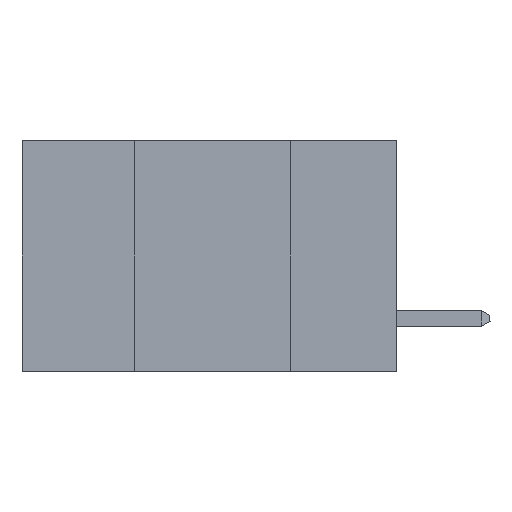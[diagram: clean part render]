
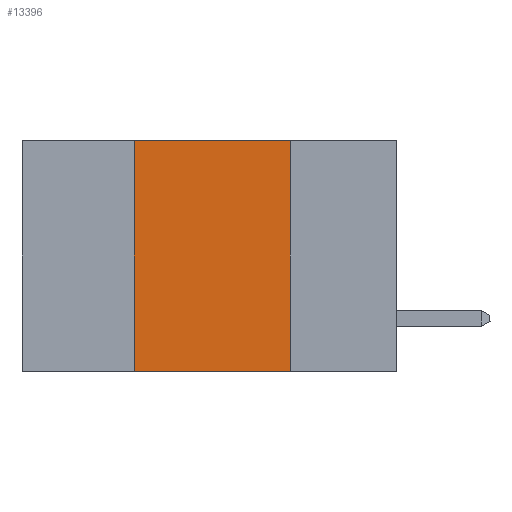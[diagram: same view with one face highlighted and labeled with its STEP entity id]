
A CAD part, left-side view. The second image highlights one B-rep face of the part: STEP entity #13396.
In plain terms, the highlighted planar face has unit normal (-1, 0, 0).
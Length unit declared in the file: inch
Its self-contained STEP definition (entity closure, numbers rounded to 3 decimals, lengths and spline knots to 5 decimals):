
#59 = LINE ( 'NONE', #626, #15693 ) ;
#314 = LINE ( 'NONE', #10184, #7683 ) ;
#399 = LINE ( 'NONE', #4879, #11413 ) ;
#626 = CARTESIAN_POINT ( 'NONE',  ( 0., 0.6, -0.37 ) ) ;
#2747 = DIRECTION ( 'NONE',  ( 0., -1., 0. ) ) ;
#3220 = CARTESIAN_POINT ( 'NONE',  ( 0., 0.42, -0.37 ) ) ;
#3722 = DIRECTION ( 'NONE',  ( 0., 0., 1. ) ) ;
#4752 = ORIENTED_EDGE ( 'NONE', *, *, #6087, .F. ) ;
#4879 = CARTESIAN_POINT ( 'NONE',  ( 0., 0.42, 0. ) ) ;
#4903 = VERTEX_POINT ( 'NONE', #10599 ) ;
#5265 = DIRECTION ( 'NONE',  ( 0., 0., -1. ) ) ;
#6087 = EDGE_CURVE ( 'NONE', #4903, #14718, #9009, .T. ) ;
#6720 = EDGE_LOOP ( 'NONE', ( #4752, #11530, #15313, #12016 ) ) ;
#7683 = VECTOR ( 'NONE', #2747, 39.37008 ) ;
#7796 = FACE_OUTER_BOUND ( 'NONE', #6720, .T. ) ;
#7815 = CARTESIAN_POINT ( 'NONE',  ( 0., 0.6, 0. ) ) ;
#8796 = CARTESIAN_POINT ( 'NONE',  ( 0., 0.17, -0.37 ) ) ;
#8860 = VERTEX_POINT ( 'NONE', #9410 ) ;
#9009 = LINE ( 'NONE', #13915, #10018 ) ;
#9224 = EDGE_CURVE ( 'NONE', #9664, #8860, #399, .T. ) ;
#9270 = DIRECTION ( 'NONE',  ( 0., -1., 0. ) ) ;
#9410 = CARTESIAN_POINT ( 'NONE',  ( 0., 0.42, 0. ) ) ;
#9664 = VERTEX_POINT ( 'NONE', #3220 ) ;
#9814 = AXIS2_PLACEMENT_3D ( 'NONE', #7815, #15173, #11510 ) ;
#10018 = VECTOR ( 'NONE', #5265, 39.37008 ) ;
#10184 = CARTESIAN_POINT ( 'NONE',  ( 0., 0.6, 0. ) ) ;
#10599 = CARTESIAN_POINT ( 'NONE',  ( 0., 0.17, 0. ) ) ;
#11131 = EDGE_CURVE ( 'NONE', #8860, #4903, #314, .T. ) ;
#11413 = VECTOR ( 'NONE', #3722, 39.37008 ) ;
#11510 = DIRECTION ( 'NONE',  ( 0., 0., -1. ) ) ;
#11530 = ORIENTED_EDGE ( 'NONE', *, *, #11131, .F. ) ;
#12016 = ORIENTED_EDGE ( 'NONE', *, *, #12785, .T. ) ;
#12749 = PLANE ( 'NONE',  #9814 ) ;
#12785 = EDGE_CURVE ( 'NONE', #9664, #14718, #59, .T. ) ;
#13396 = ADVANCED_FACE ( 'NONE', ( #7796 ), #12749, .F. ) ;
#13915 = CARTESIAN_POINT ( 'NONE',  ( 0., 0.17, 0. ) ) ;
#14718 = VERTEX_POINT ( 'NONE', #8796 ) ;
#15173 = DIRECTION ( 'NONE',  ( 1., 0., 0. ) ) ;
#15313 = ORIENTED_EDGE ( 'NONE', *, *, #9224, .F. ) ;
#15693 = VECTOR ( 'NONE', #9270, 39.37008 ) ;
